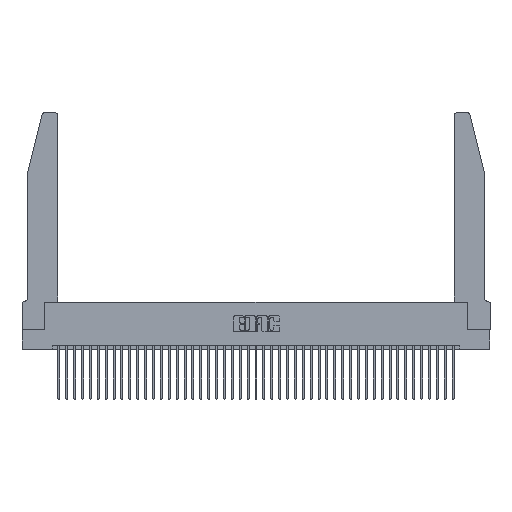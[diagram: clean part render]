
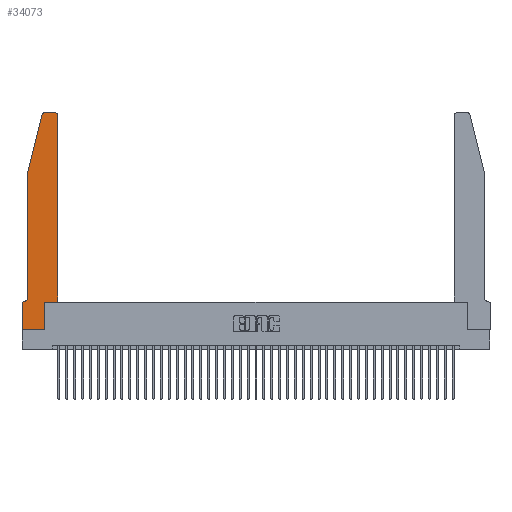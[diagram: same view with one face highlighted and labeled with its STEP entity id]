
A CAD part, top view. The second image highlights one B-rep face of the part: STEP entity #34073.
In plain terms, the highlighted planar face has unit normal (0, 0, 1).
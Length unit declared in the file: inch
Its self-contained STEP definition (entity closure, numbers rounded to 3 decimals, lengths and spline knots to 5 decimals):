
#542 = VERTEX_POINT ( 'NONE', #29179 ) ;
#770 = ORIENTED_EDGE ( 'NONE', *, *, #39346, .T. ) ;
#1034 = EDGE_CURVE ( 'NONE', #36491, #26967, #2297, .T. ) ;
#1061 = LINE ( 'NONE', #43096, #18473 ) ;
#1287 = CARTESIAN_POINT ( 'NONE',  ( 0., 0.35, 0.37 ) ) ;
#2252 = EDGE_CURVE ( 'NONE', #31250, #542, #12217, .T. ) ;
#2297 = CIRCLE ( 'NONE', #36681, 0.03 ) ;
#2449 = AXIS2_PLACEMENT_3D ( 'NONE', #23817, #30562, #10055 ) ;
#3844 = CARTESIAN_POINT ( 'NONE',  ( 0.2865, 0., 0.37 ) ) ;
#3932 = VERTEX_POINT ( 'NONE', #33291 ) ;
#4051 = VERTEX_POINT ( 'NONE', #17809 ) ;
#4602 = DIRECTION ( 'NONE',  ( 0., 0., -1. ) ) ;
#5462 = EDGE_CURVE ( 'NONE', #4051, #3932, #1061, .T. ) ;
#5833 = VECTOR ( 'NONE', #27454, 39.37008 ) ;
#7098 = CARTESIAN_POINT ( 'NONE',  ( 0.4505, 0.35, 0.37 ) ) ;
#7127 = CIRCLE ( 'NONE', #34647, 0.07 ) ;
#8294 = CARTESIAN_POINT ( 'NONE',  ( 0.4505, 0.35, 0.37 ) ) ;
#9945 = DIRECTION ( 'NONE',  ( 1., 0., 0. ) ) ;
#9950 = ORIENTED_EDGE ( 'NONE', *, *, #24443, .T. ) ;
#10055 = DIRECTION ( 'NONE',  ( 1., 0., 0. ) ) ;
#10315 = VECTOR ( 'NONE', #9945, 39.37008 ) ;
#11069 = LINE ( 'NONE', #14005, #24821 ) ;
#11581 = VERTEX_POINT ( 'NONE', #42456 ) ;
#12119 = CARTESIAN_POINT ( 'NONE',  ( 0.2605, 2.75, 0.37 ) ) ;
#12217 = LINE ( 'NONE', #13880, #5833 ) ;
#12827 = LINE ( 'NONE', #12119, #29207 ) ;
#13498 = DIRECTION ( 'NONE',  ( -0.239, -0.971, 0. ) ) ;
#13880 = CARTESIAN_POINT ( 'NONE',  ( 0.0755, 2., 0.37 ) ) ;
#13934 = CARTESIAN_POINT ( 'NONE',  ( 0.0755, 2., 0.37 ) ) ;
#14005 = CARTESIAN_POINT ( 'NONE',  ( 0.0755, 0.35, 0.37 ) ) ;
#14951 = EDGE_CURVE ( 'NONE', #3932, #34470, #32612, .T. ) ;
#14996 = DIRECTION ( 'NONE',  ( 0., 0., 1. ) ) ;
#15176 = CARTESIAN_POINT ( 'NONE',  ( 0.4505, 0.35, 0.37 ) ) ;
#15999 = CARTESIAN_POINT ( 'NONE',  ( 0.4505, 2.72, 0.37 ) ) ;
#16308 = LINE ( 'NONE', #15176, #35269 ) ;
#16761 = DIRECTION ( 'NONE',  ( 0., 1., 0. ) ) ;
#17291 = VERTEX_POINT ( 'NONE', #8294 ) ;
#17337 = VERTEX_POINT ( 'NONE', #17534 ) ;
#17534 = CARTESIAN_POINT ( 'NONE',  ( 0.25487, 2.72718, 0.37 ) ) ;
#17809 = CARTESIAN_POINT ( 'NONE',  ( 0., 0.35, 0.37 ) ) ;
#18324 = ORIENTED_EDGE ( 'NONE', *, *, #21622, .T. ) ;
#18473 = VECTOR ( 'NONE', #36760, 39.37008 ) ;
#18596 = DIRECTION ( 'NONE',  ( 0., 1., 0. ) ) ;
#18694 = CARTESIAN_POINT ( 'NONE',  ( 0.0055, 0.35, 0.37 ) ) ;
#19031 = AXIS2_PLACEMENT_3D ( 'NONE', #1287, #14996, #38682 ) ;
#19299 = CARTESIAN_POINT ( 'NONE',  ( 0.2865, 0.35, 0.37 ) ) ;
#19366 = VECTOR ( 'NONE', #13498, 39.37008 ) ;
#19827 = VERTEX_POINT ( 'NONE', #23898 ) ;
#20026 = VECTOR ( 'NONE', #16761, 39.37008 ) ;
#21622 = EDGE_CURVE ( 'NONE', #34470, #11581, #30007, .T. ) ;
#23523 = EDGE_CURVE ( 'NONE', #17337, #31250, #43013, .T. ) ;
#23544 = EDGE_CURVE ( 'NONE', #11581, #17291, #36154, .T. ) ;
#23651 = VERTEX_POINT ( 'NONE', #18694 ) ;
#23817 = CARTESIAN_POINT ( 'NONE',  ( 0.284, 2.72, 0.37 ) ) ;
#23898 = CARTESIAN_POINT ( 'NONE',  ( 0.284, 2.75, 0.37 ) ) ;
#23954 = CARTESIAN_POINT ( 'NONE',  ( 0.4205, 2.75, 0.37 ) ) ;
#23968 = CARTESIAN_POINT ( 'NONE',  ( 0.4205, 2.72, 0.37 ) ) ;
#24264 = ORIENTED_EDGE ( 'NONE', *, *, #23544, .T. ) ;
#24443 = EDGE_CURVE ( 'NONE', #542, #23651, #7127, .T. ) ;
#24821 = VECTOR ( 'NONE', #27423, 39.37008 ) ;
#24869 = CARTESIAN_POINT ( 'NONE',  ( 0.0055, 0.42, 0.37 ) ) ;
#25728 = ORIENTED_EDGE ( 'NONE', *, *, #25930, .T. ) ;
#25930 = EDGE_CURVE ( 'NONE', #26967, #19827, #12827, .T. ) ;
#26196 = DIRECTION ( 'NONE',  ( 1., 0., 0. ) ) ;
#26247 = ORIENTED_EDGE ( 'NONE', *, *, #28236, .T. ) ;
#26757 = EDGE_LOOP ( 'NONE', ( #25728, #770, #42162, #42809, #9950, #41470, #36646, #32832, #18324, #24264, #26247, #42572 ) ) ;
#26967 = VERTEX_POINT ( 'NONE', #23954 ) ;
#27423 = DIRECTION ( 'NONE',  ( -1., 0., 0. ) ) ;
#27454 = DIRECTION ( 'NONE',  ( 0., -1., 0. ) ) ;
#27472 = DIRECTION ( 'NONE',  ( 1., 0., 0. ) ) ;
#28236 = EDGE_CURVE ( 'NONE', #17291, #36491, #16308, .T. ) ;
#29179 = CARTESIAN_POINT ( 'NONE',  ( 0.0755, 0.42, 0.37 ) ) ;
#29207 = VECTOR ( 'NONE', #33070, 39.37008 ) ;
#30007 = LINE ( 'NONE', #19299, #20026 ) ;
#30562 = DIRECTION ( 'NONE',  ( 0., 0., 1. ) ) ;
#31250 = VERTEX_POINT ( 'NONE', #40964 ) ;
#31615 = DIRECTION ( 'NONE',  ( -1., 0., 0. ) ) ;
#32076 = PLANE ( 'NONE',  #19031 ) ;
#32612 = LINE ( 'NONE', #43511, #34698 ) ;
#32832 = ORIENTED_EDGE ( 'NONE', *, *, #14951, .T. ) ;
#33070 = DIRECTION ( 'NONE',  ( -1., 0., 0. ) ) ;
#33274 = EDGE_CURVE ( 'NONE', #23651, #4051, #11069, .T. ) ;
#33291 = CARTESIAN_POINT ( 'NONE',  ( 0., 0., 0.37 ) ) ;
#34073 = ADVANCED_FACE ( 'NONE', ( #34196 ), #32076, .T. ) ;
#34196 = FACE_OUTER_BOUND ( 'NONE', #26757, .T. ) ;
#34470 = VERTEX_POINT ( 'NONE', #3844 ) ;
#34647 = AXIS2_PLACEMENT_3D ( 'NONE', #24869, #4602, #31615 ) ;
#34698 = VECTOR ( 'NONE', #26196, 39.37008 ) ;
#35269 = VECTOR ( 'NONE', #18596, 39.37008 ) ;
#36154 = LINE ( 'NONE', #7098, #10315 ) ;
#36336 = CIRCLE ( 'NONE', #2449, 0.03 ) ;
#36491 = VERTEX_POINT ( 'NONE', #15999 ) ;
#36646 = ORIENTED_EDGE ( 'NONE', *, *, #5462, .T. ) ;
#36681 = AXIS2_PLACEMENT_3D ( 'NONE', #23968, #41118, #27472 ) ;
#36760 = DIRECTION ( 'NONE',  ( 0., -1., 0. ) ) ;
#38682 = DIRECTION ( 'NONE',  ( 1., 0., 0. ) ) ;
#39346 = EDGE_CURVE ( 'NONE', #19827, #17337, #36336, .T. ) ;
#40964 = CARTESIAN_POINT ( 'NONE',  ( 0.0755, 2., 0.37 ) ) ;
#41118 = DIRECTION ( 'NONE',  ( 0., 0., 1. ) ) ;
#41470 = ORIENTED_EDGE ( 'NONE', *, *, #33274, .T. ) ;
#42162 = ORIENTED_EDGE ( 'NONE', *, *, #23523, .T. ) ;
#42456 = CARTESIAN_POINT ( 'NONE',  ( 0.2865, 0.35, 0.37 ) ) ;
#42572 = ORIENTED_EDGE ( 'NONE', *, *, #1034, .T. ) ;
#42809 = ORIENTED_EDGE ( 'NONE', *, *, #2252, .T. ) ;
#43013 = LINE ( 'NONE', #13934, #19366 ) ;
#43096 = CARTESIAN_POINT ( 'NONE',  ( 0., 0., 0.37 ) ) ;
#43511 = CARTESIAN_POINT ( 'NONE',  ( 0., 0., 0.37 ) ) ;
